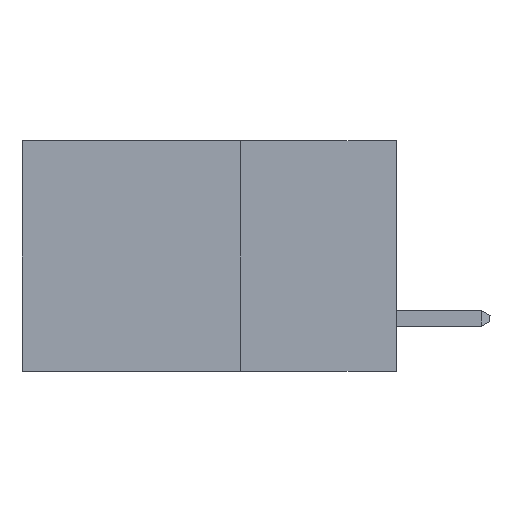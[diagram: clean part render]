
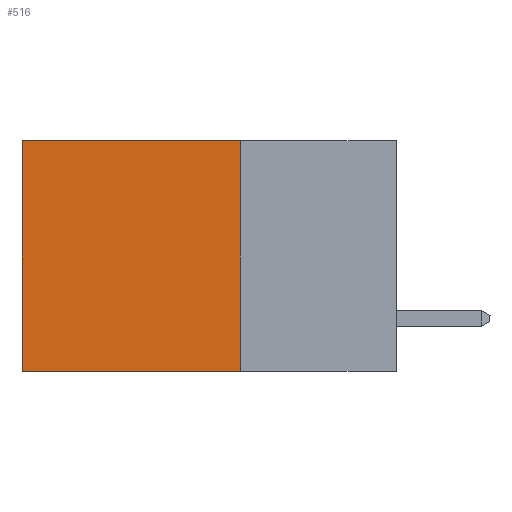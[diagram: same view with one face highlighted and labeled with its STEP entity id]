
A CAD part, left-side view. The second image highlights one B-rep face of the part: STEP entity #516.
In plain terms, the highlighted planar face has unit normal (-1, 0, 0).
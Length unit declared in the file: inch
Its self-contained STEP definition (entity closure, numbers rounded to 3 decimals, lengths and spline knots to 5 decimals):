
#231 = VERTEX_POINT ( 'NONE', #4262 ) ;
#516 = ADVANCED_FACE ( 'NONE', ( #5883 ), #10553, .F. ) ;
#626 = CARTESIAN_POINT ( 'NONE',  ( 0.2615, 0.25, 0. ) ) ;
#638 = DIRECTION ( 'NONE',  ( 0., 0., -1. ) ) ;
#2098 = VECTOR ( 'NONE', #5579, 39.37008 ) ;
#2115 = LINE ( 'NONE', #626, #10563 ) ;
#2125 = EDGE_CURVE ( 'NONE', #6347, #231, #2115, .T. ) ;
#2312 = LINE ( 'NONE', #3823, #4763 ) ;
#2447 = DIRECTION ( 'NONE',  ( 0., 1., 0. ) ) ;
#2969 = VERTEX_POINT ( 'NONE', #7684 ) ;
#3267 = EDGE_LOOP ( 'NONE', ( #4801, #4526, #3645, #6094 ) ) ;
#3600 = VERTEX_POINT ( 'NONE', #8182 ) ;
#3645 = ORIENTED_EDGE ( 'NONE', *, *, #7563, .F. ) ;
#3823 = CARTESIAN_POINT ( 'NONE',  ( 0.2615, 0.25, -0.37 ) ) ;
#3925 = DIRECTION ( 'NONE',  ( 0., 0., -1. ) ) ;
#4092 = VECTOR ( 'NONE', #638, 39.37008 ) ;
#4262 = CARTESIAN_POINT ( 'NONE',  ( 0.2615, 0.6, 0. ) ) ;
#4526 = ORIENTED_EDGE ( 'NONE', *, *, #9716, .F. ) ;
#4763 = VECTOR ( 'NONE', #10354, 39.37008 ) ;
#4769 = CARTESIAN_POINT ( 'NONE',  ( 0.2615, 0.25, -0.37 ) ) ;
#4801 = ORIENTED_EDGE ( 'NONE', *, *, #6259, .T. ) ;
#4911 = DIRECTION ( 'NONE',  ( 1., 0., 0. ) ) ;
#5579 = DIRECTION ( 'NONE',  ( 0., 0., -1. ) ) ;
#5883 = FACE_OUTER_BOUND ( 'NONE', #3267, .T. ) ;
#6094 = ORIENTED_EDGE ( 'NONE', *, *, #2125, .T. ) ;
#6259 = EDGE_CURVE ( 'NONE', #231, #3600, #7891, .T. ) ;
#6347 = VERTEX_POINT ( 'NONE', #9093 ) ;
#6472 = LINE ( 'NONE', #4769, #2098 ) ;
#7563 = EDGE_CURVE ( 'NONE', #6347, #2969, #6472, .T. ) ;
#7684 = CARTESIAN_POINT ( 'NONE',  ( 0.2615, 0.25, -0.37 ) ) ;
#7891 = LINE ( 'NONE', #10532, #4092 ) ;
#7907 = CARTESIAN_POINT ( 'NONE',  ( 0.2615, 0.25, -0.37 ) ) ;
#8182 = CARTESIAN_POINT ( 'NONE',  ( 0.2615, 0.6, -0.37 ) ) ;
#9077 = AXIS2_PLACEMENT_3D ( 'NONE', #7907, #4911, #3925 ) ;
#9093 = CARTESIAN_POINT ( 'NONE',  ( 0.2615, 0.25, 0. ) ) ;
#9716 = EDGE_CURVE ( 'NONE', #2969, #3600, #2312, .T. ) ;
#10354 = DIRECTION ( 'NONE',  ( 0., 1., 0. ) ) ;
#10532 = CARTESIAN_POINT ( 'NONE',  ( 0.2615, 0.6, -0.37 ) ) ;
#10553 = PLANE ( 'NONE',  #9077 ) ;
#10563 = VECTOR ( 'NONE', #2447, 39.37008 ) ;
